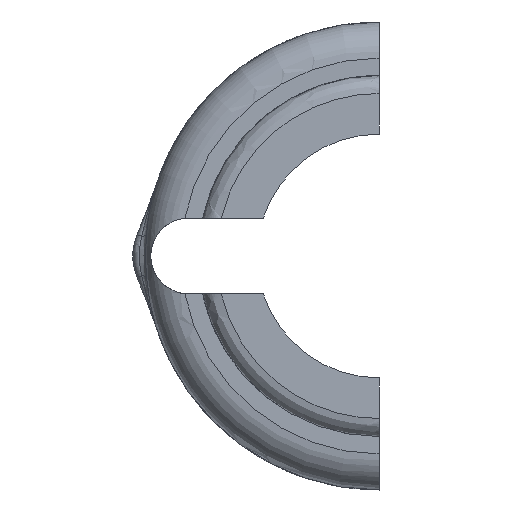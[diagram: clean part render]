
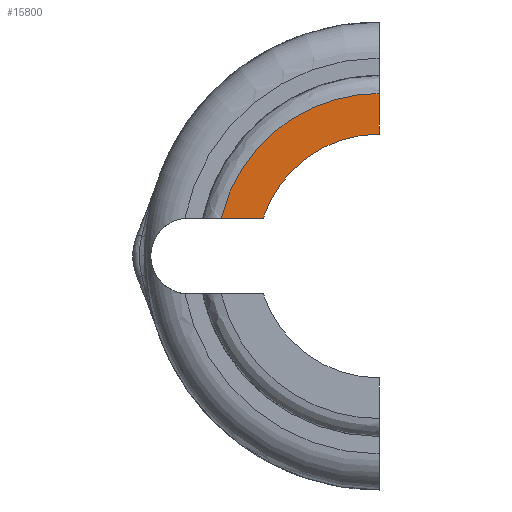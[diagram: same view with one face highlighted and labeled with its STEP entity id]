
A CAD part, left-side view. The second image highlights one B-rep face of the part: STEP entity #15800.
In plain terms, the highlighted planar face has unit normal (-1, 0, 0).
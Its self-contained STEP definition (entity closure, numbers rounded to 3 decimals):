
#211 = EDGE_CURVE ( 'NONE', #23298, #55765, #33822, .T. ) ;
#3310 = PLANE ( 'NONE',  #31734 ) ;
#3998 = VERTEX_POINT ( 'NONE', #49121 ) ;
#5707 = EDGE_CURVE ( 'NONE', #55765, #21696, #46154, .T. ) ;
#8665 = FACE_OUTER_BOUND ( 'NONE', #17725, .T. ) ;
#11056 = EDGE_CURVE ( 'NONE', #3998, #23298, #58868, .T. ) ;
#11739 = DIRECTION ( 'NONE',  ( 1., 0., 0. ) ) ;
#14744 = CARTESIAN_POINT ( 'NONE',  ( -170., 8.652, 18. ) ) ;
#14904 = CARTESIAN_POINT ( 'NONE',  ( -170., 0., 13.5 ) ) ;
#15133 = ORIENTED_EDGE ( 'NONE', *, *, #5707, .T. ) ;
#15800 = ADVANCED_FACE ( 'NONE', ( #8665 ), #3310, .T. ) ;
#16122 = AXIS2_PLACEMENT_3D ( 'NONE', #49999, #11739, #60629 ) ;
#17390 = VECTOR ( 'NONE', #40887, 1000. ) ;
#17575 = CARTESIAN_POINT ( 'NONE',  ( -170., 8.804, 4.2 ) ) ;
#17725 = EDGE_LOOP ( 'NONE', ( #15133, #54337, #52959, #36890 ) ) ;
#21696 = VERTEX_POINT ( 'NONE', #60345 ) ;
#23298 = VERTEX_POINT ( 'NONE', #31028 ) ;
#25300 = DIRECTION ( 'NONE',  ( -1., 0., 0. ) ) ;
#31028 = CARTESIAN_POINT ( 'NONE',  ( -170., 12.83, 4.2 ) ) ;
#31342 =( BOUNDED_CURVE ( )  B_SPLINE_CURVE ( 3, ( #41696, #41236, #14744, #52543 ),
 .UNSPECIFIED., .F., .T. ) 
 B_SPLINE_CURVE_WITH_KNOTS ( ( 4, 4 ),
 ( 0., 1. ),
 .UNSPECIFIED. ) 
 CURVE ( )  GEOMETRIC_REPRESENTATION_ITEM ( )  RATIONAL_B_SPLINE_CURVE ( ( 0.989, 0.85, 0.854, 1. ) ) 
 REPRESENTATION_ITEM ( '' )  );
#31734 = AXIS2_PLACEMENT_3D ( 'NONE', #57684, #25300, #63085 ) ;
#33822 = CIRCLE ( 'NONE', #16122, 13.5 ) ;
#35442 = CARTESIAN_POINT ( 'NONE',  ( -170., 0., 20.747 ) ) ;
#36890 = ORIENTED_EDGE ( 'NONE', *, *, #211, .T. ) ;
#40887 = DIRECTION ( 'NONE',  ( 0., 0., 1. ) ) ;
#41236 = CARTESIAN_POINT ( 'NONE',  ( -170., 15.476, 12.65 ) ) ;
#41696 = CARTESIAN_POINT ( 'NONE',  ( -170., 17.503, 4.2 ) ) ;
#42358 = EDGE_CURVE ( 'NONE', #3998, #21696, #31342, .T. ) ;
#46154 = LINE ( 'NONE', #35442, #17390 ) ;
#46202 = VECTOR ( 'NONE', #61047, 1000. ) ;
#49121 = CARTESIAN_POINT ( 'NONE',  ( -170., 17.503, 4.2 ) ) ;
#49999 = CARTESIAN_POINT ( 'NONE',  ( -170., 0., 0. ) ) ;
#52543 = CARTESIAN_POINT ( 'NONE',  ( -170., 0., 18. ) ) ;
#52959 = ORIENTED_EDGE ( 'NONE', *, *, #11056, .T. ) ;
#54337 = ORIENTED_EDGE ( 'NONE', *, *, #42358, .F. ) ;
#55765 = VERTEX_POINT ( 'NONE', #14904 ) ;
#57684 = CARTESIAN_POINT ( 'NONE',  ( -170., 17.608, 18.083 ) ) ;
#58868 = LINE ( 'NONE', #17575, #46202 ) ;
#60345 = CARTESIAN_POINT ( 'NONE',  ( -170., 0., 18. ) ) ;
#60629 = DIRECTION ( 'NONE',  ( 0., -1., 0. ) ) ;
#61047 = DIRECTION ( 'NONE',  ( 0., -1., 0. ) ) ;
#63085 = DIRECTION ( 'NONE',  ( 0., 0., -1. ) ) ;
